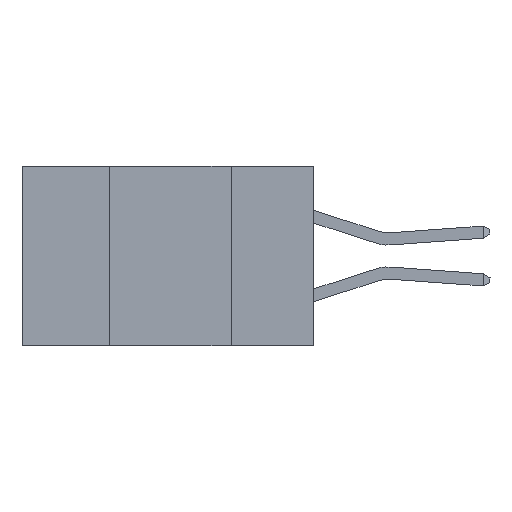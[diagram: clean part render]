
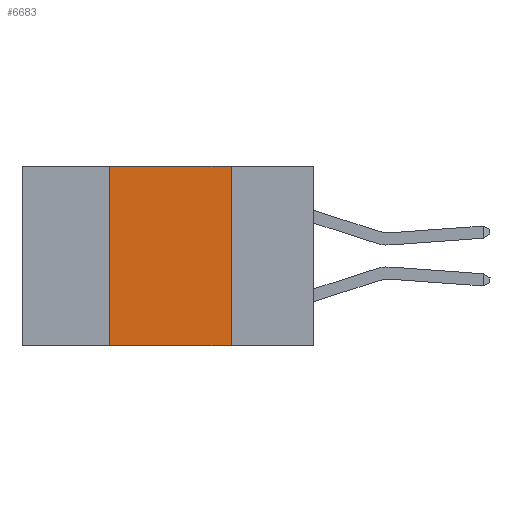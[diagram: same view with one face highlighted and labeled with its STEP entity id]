
A CAD part, left-side view. The second image highlights one B-rep face of the part: STEP entity #6683.
In plain terms, the highlighted planar face has unit normal (-1, 0, 0).
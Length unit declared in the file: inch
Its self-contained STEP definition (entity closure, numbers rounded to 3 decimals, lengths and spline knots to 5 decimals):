
#1037 = CARTESIAN_POINT ( 'NONE',  ( 0., 0.6, 0. ) ) ;
#1178 = VECTOR ( 'NONE', #4707, 39.37008 ) ;
#1758 = LINE ( 'NONE', #16469, #11827 ) ;
#2039 = ORIENTED_EDGE ( 'NONE', *, *, #23412, .T. ) ;
#3904 = LINE ( 'NONE', #14881, #21507 ) ;
#4707 = DIRECTION ( 'NONE',  ( 0., -1., 0. ) ) ;
#4896 = DIRECTION ( 'NONE',  ( 0., 0., -1. ) ) ;
#5573 = DIRECTION ( 'NONE',  ( 0., -1., 0. ) ) ;
#6683 = ADVANCED_FACE ( 'NONE', ( #7047 ), #12067, .F. ) ;
#7047 = FACE_OUTER_BOUND ( 'NONE', #23445, .T. ) ;
#7093 = EDGE_CURVE ( 'NONE', #23314, #11105, #9086, .T. ) ;
#8617 = DIRECTION ( 'NONE',  ( 0., 0., -1. ) ) ;
#8805 = ORIENTED_EDGE ( 'NONE', *, *, #7093, .F. ) ;
#9086 = LINE ( 'NONE', #23531, #21073 ) ;
#9140 = CARTESIAN_POINT ( 'NONE',  ( 0., 0.42, -0.37 ) ) ;
#9721 = CARTESIAN_POINT ( 'NONE',  ( 0., 0.17, 0. ) ) ;
#10647 = AXIS2_PLACEMENT_3D ( 'NONE', #1037, #20113, #8617 ) ;
#11105 = VERTEX_POINT ( 'NONE', #23849 ) ;
#11827 = VECTOR ( 'NONE', #4896, 39.37008 ) ;
#11946 = VERTEX_POINT ( 'NONE', #9721 ) ;
#12067 = PLANE ( 'NONE',  #10647 ) ;
#12193 = ORIENTED_EDGE ( 'NONE', *, *, #23784, .F. ) ;
#14881 = CARTESIAN_POINT ( 'NONE',  ( 0., 0.6, -0.37 ) ) ;
#15261 = VERTEX_POINT ( 'NONE', #23581 ) ;
#16041 = LINE ( 'NONE', #16106, #1178 ) ;
#16106 = CARTESIAN_POINT ( 'NONE',  ( 0., 0.6, 0. ) ) ;
#16469 = CARTESIAN_POINT ( 'NONE',  ( 0., 0.17, 0. ) ) ;
#16609 = EDGE_CURVE ( 'NONE', #11946, #15261, #1758, .T. ) ;
#19781 = DIRECTION ( 'NONE',  ( 0., 0., 1. ) ) ;
#20113 = DIRECTION ( 'NONE',  ( 1., 0., 0. ) ) ;
#20772 = ORIENTED_EDGE ( 'NONE', *, *, #16609, .F. ) ;
#21073 = VECTOR ( 'NONE', #19781, 39.37008 ) ;
#21507 = VECTOR ( 'NONE', #5573, 39.37008 ) ;
#23314 = VERTEX_POINT ( 'NONE', #9140 ) ;
#23412 = EDGE_CURVE ( 'NONE', #23314, #15261, #3904, .T. ) ;
#23445 = EDGE_LOOP ( 'NONE', ( #20772, #12193, #8805, #2039 ) ) ;
#23531 = CARTESIAN_POINT ( 'NONE',  ( 0., 0.42, 0. ) ) ;
#23581 = CARTESIAN_POINT ( 'NONE',  ( 0., 0.17, -0.37 ) ) ;
#23784 = EDGE_CURVE ( 'NONE', #11105, #11946, #16041, .T. ) ;
#23849 = CARTESIAN_POINT ( 'NONE',  ( 0., 0.42, 0. ) ) ;
